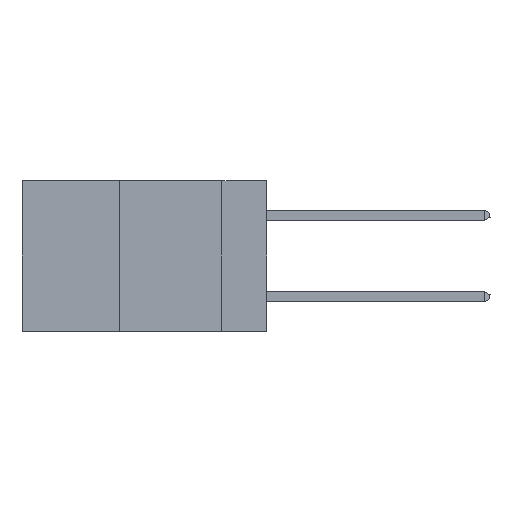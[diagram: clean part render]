
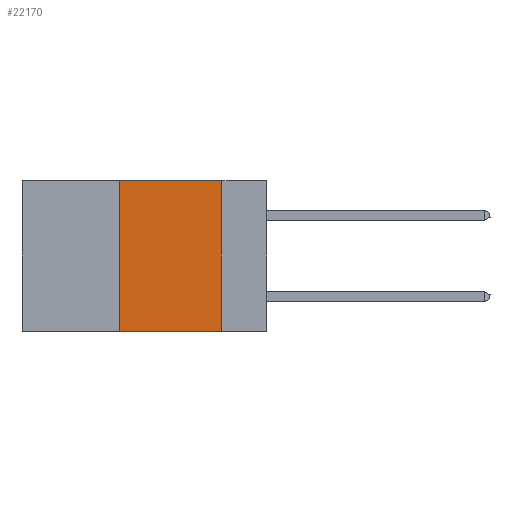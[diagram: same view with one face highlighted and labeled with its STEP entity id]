
A CAD part, left-side view. The second image highlights one B-rep face of the part: STEP entity #22170.
In plain terms, the highlighted planar face has unit normal (-1, 0, 0).
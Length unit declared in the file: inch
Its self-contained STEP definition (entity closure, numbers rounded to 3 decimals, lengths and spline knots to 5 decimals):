
#37 = AXIS2_PLACEMENT_3D ( 'NONE', #30435, #33945, #17057 ) ;
#112 = CARTESIAN_POINT ( 'NONE',  ( 0., 0.36, -0.37 ) ) ;
#1579 = CARTESIAN_POINT ( 'NONE',  ( 0., 0.11, -0.37 ) ) ;
#2208 = LINE ( 'NONE', #31534, #20063 ) ;
#2408 = ORIENTED_EDGE ( 'NONE', *, *, #40897, .F. ) ;
#2974 = ORIENTED_EDGE ( 'NONE', *, *, #37441, .F. ) ;
#3858 = VERTEX_POINT ( 'NONE', #1579 ) ;
#5714 = DIRECTION ( 'NONE',  ( 0., -1., 0. ) ) ;
#7121 = CARTESIAN_POINT ( 'NONE',  ( 0., 0.6, 0. ) ) ;
#7987 = EDGE_LOOP ( 'NONE', ( #2408, #2974, #16676, #26003 ) ) ;
#12294 = LINE ( 'NONE', #15629, #35443 ) ;
#15629 = CARTESIAN_POINT ( 'NONE',  ( 0., 0.36, 0. ) ) ;
#16123 = CARTESIAN_POINT ( 'NONE',  ( 0., 0.11, 0. ) ) ;
#16676 = ORIENTED_EDGE ( 'NONE', *, *, #39711, .F. ) ;
#17057 = DIRECTION ( 'NONE',  ( 0., 0., -1. ) ) ;
#17137 = DIRECTION ( 'NONE',  ( 0., -1., 0. ) ) ;
#20063 = VECTOR ( 'NONE', #31679, 39.37008 ) ;
#22170 = ADVANCED_FACE ( 'NONE', ( #38363 ), #23212, .F. ) ;
#22374 = DIRECTION ( 'NONE',  ( 0., 0., 1. ) ) ;
#23212 = PLANE ( 'NONE',  #37 ) ;
#24904 = EDGE_CURVE ( 'NONE', #37369, #3858, #42236, .T. ) ;
#26003 = ORIENTED_EDGE ( 'NONE', *, *, #24904, .T. ) ;
#30435 = CARTESIAN_POINT ( 'NONE',  ( 0., 0.6, 0. ) ) ;
#31534 = CARTESIAN_POINT ( 'NONE',  ( 0., 0.11, 0. ) ) ;
#31679 = DIRECTION ( 'NONE',  ( 0., 0., -1. ) ) ;
#33120 = VERTEX_POINT ( 'NONE', #16123 ) ;
#33945 = DIRECTION ( 'NONE',  ( 1., 0., 0. ) ) ;
#34061 = CARTESIAN_POINT ( 'NONE',  ( 0., 0.36, 0. ) ) ;
#34659 = VERTEX_POINT ( 'NONE', #34061 ) ;
#35443 = VECTOR ( 'NONE', #22374, 39.37008 ) ;
#37369 = VERTEX_POINT ( 'NONE', #112 ) ;
#37441 = EDGE_CURVE ( 'NONE', #34659, #33120, #37677, .T. ) ;
#37677 = LINE ( 'NONE', #7121, #38707 ) ;
#38067 = VECTOR ( 'NONE', #5714, 39.37008 ) ;
#38363 = FACE_OUTER_BOUND ( 'NONE', #7987, .T. ) ;
#38707 = VECTOR ( 'NONE', #17137, 39.37008 ) ;
#39711 = EDGE_CURVE ( 'NONE', #37369, #34659, #12294, .T. ) ;
#40897 = EDGE_CURVE ( 'NONE', #33120, #3858, #2208, .T. ) ;
#42236 = LINE ( 'NONE', #42819, #38067 ) ;
#42819 = CARTESIAN_POINT ( 'NONE',  ( 0., 0.6, -0.37 ) ) ;
